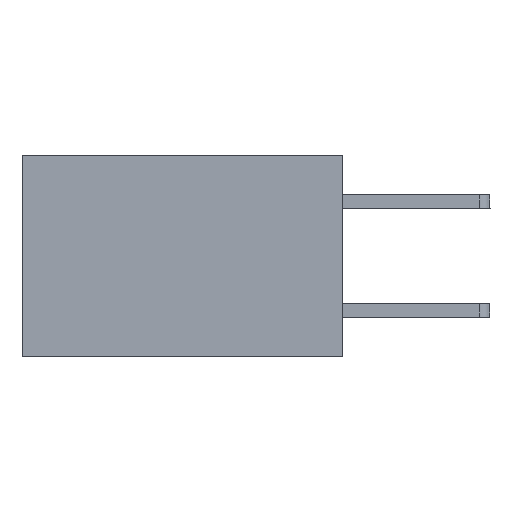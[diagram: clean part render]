
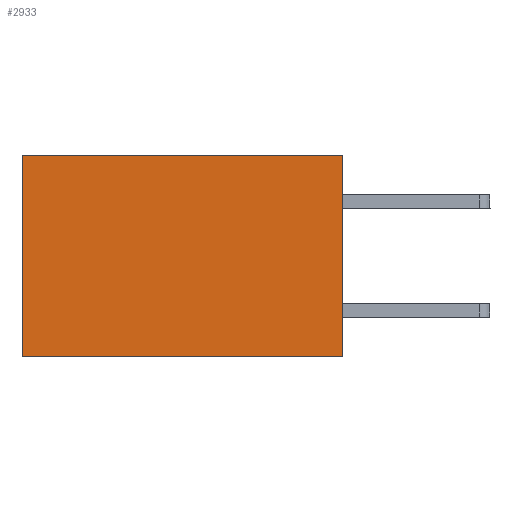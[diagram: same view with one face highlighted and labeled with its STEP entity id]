
A CAD part, left-side view. The second image highlights one B-rep face of the part: STEP entity #2933.
In plain terms, the highlighted planar face has unit normal (-1, 0, 0).
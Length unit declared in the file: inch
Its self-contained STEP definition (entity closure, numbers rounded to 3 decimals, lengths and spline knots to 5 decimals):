
#165 = ORIENTED_EDGE ( 'NONE', *, *, #4776, .T. ) ;
#226 = EDGE_LOOP ( 'NONE', ( #165, #3013, #549, #8755 ) ) ;
#476 = LINE ( 'NONE', #4953, #4428 ) ;
#549 = ORIENTED_EDGE ( 'NONE', *, *, #876, .F. ) ;
#851 = LINE ( 'NONE', #4863, #3785 ) ;
#858 = EDGE_CURVE ( 'NONE', #1818, #8213, #851, .T. ) ;
#876 = EDGE_CURVE ( 'NONE', #8071, #1818, #476, .T. ) ;
#1818 = VERTEX_POINT ( 'NONE', #9351 ) ;
#2408 = DIRECTION ( 'NONE',  ( 0., 1., 0. ) ) ;
#2933 = ADVANCED_FACE ( 'NONE', ( #11316 ), #5131, .F. ) ;
#3013 = ORIENTED_EDGE ( 'NONE', *, *, #858, .F. ) ;
#3079 = EDGE_CURVE ( 'NONE', #8071, #3658, #6944, .T. ) ;
#3110 = VECTOR ( 'NONE', #10563, 39.37008 ) ;
#3360 = DIRECTION ( 'NONE',  ( 0., 1., 0. ) ) ;
#3404 = CARTESIAN_POINT ( 'NONE',  ( 0.277, 0., 0. ) ) ;
#3638 = CARTESIAN_POINT ( 'NONE',  ( 0.277, 0.59, 0. ) ) ;
#3654 = DIRECTION ( 'NONE',  ( 0., 0., -1. ) ) ;
#3658 = VERTEX_POINT ( 'NONE', #3638 ) ;
#3785 = VECTOR ( 'NONE', #2408, 39.37008 ) ;
#4428 = VECTOR ( 'NONE', #3654, 39.37008 ) ;
#4751 = VECTOR ( 'NONE', #3360, 39.37008 ) ;
#4776 = EDGE_CURVE ( 'NONE', #3658, #8213, #9678, .T. ) ;
#4863 = CARTESIAN_POINT ( 'NONE',  ( 0.277, 0., -0.37 ) ) ;
#4893 = CARTESIAN_POINT ( 'NONE',  ( 0.277, 0.59, -0.37 ) ) ;
#4953 = CARTESIAN_POINT ( 'NONE',  ( 0.277, 0., -0.37 ) ) ;
#4997 = DIRECTION ( 'NONE',  ( 0., 0., -1. ) ) ;
#5003 = DIRECTION ( 'NONE',  ( 1., 0., 0. ) ) ;
#5044 = CARTESIAN_POINT ( 'NONE',  ( 0.277, 0., -0.37 ) ) ;
#5131 = PLANE ( 'NONE',  #6607 ) ;
#6429 = CARTESIAN_POINT ( 'NONE',  ( 0.277, 0.59, -0.37 ) ) ;
#6607 = AXIS2_PLACEMENT_3D ( 'NONE', #5044, #5003, #4997 ) ;
#6944 = LINE ( 'NONE', #3404, #4751 ) ;
#7177 = CARTESIAN_POINT ( 'NONE',  ( 0.277, 0., 0. ) ) ;
#8071 = VERTEX_POINT ( 'NONE', #7177 ) ;
#8213 = VERTEX_POINT ( 'NONE', #6429 ) ;
#8755 = ORIENTED_EDGE ( 'NONE', *, *, #3079, .T. ) ;
#9351 = CARTESIAN_POINT ( 'NONE',  ( 0.277, 0., -0.37 ) ) ;
#9678 = LINE ( 'NONE', #4893, #3110 ) ;
#10563 = DIRECTION ( 'NONE',  ( 0., 0., -1. ) ) ;
#11316 = FACE_OUTER_BOUND ( 'NONE', #226, .T. ) ;
